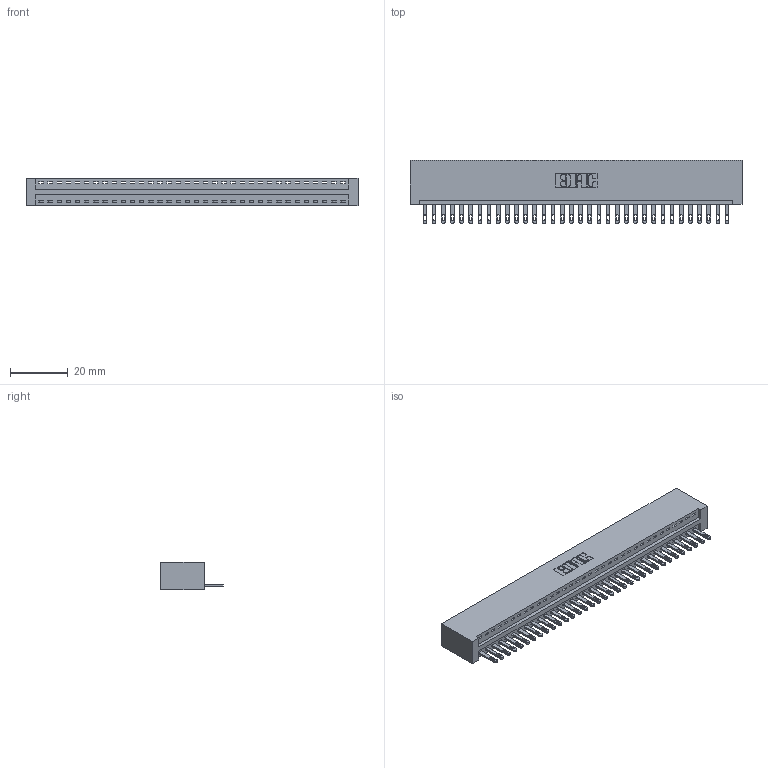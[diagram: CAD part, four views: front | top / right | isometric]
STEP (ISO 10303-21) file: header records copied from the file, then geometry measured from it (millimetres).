
FILE_DESCRIPTION (( 'STEP AP203' ), '1' );
FILE_NAME ('346-034-500-101.STEP', '2022-05-06T20:37:02', ( '' ), ( '' ), 'SwSTEP 2.0', 'SolidWorks 2020', '' );
FILE_SCHEMA (( 'CONFIG_CONTROL_DESIGN' ));
Length unit declared in the file: inch
Products named in the file (3): 346 Part_No Mounting Lugs; 345-292-001_345-293-100; 346-034-500-101
Assembly tree (35 placements, depth 2):
  346-034-500-101
    346 Part_No Mounting Lugs
    345-292-001_345-293-100  x34
Bounding box: 115.19 x 21.84 x 9.4 mm (x, y, z)
Volume: 11541.5 mm3; surface area: 14493.4 mm2
Topology: 35 solids, 35 shells, 1950 faces, 6017 edges, 4010 vertices
Faces by surface type: plane 1228, cylinder 722
Entity records: 21831 total; most frequent: CARTESIAN_POINT 3750, ORIENTED_EDGE 3718, DIRECTION 3315, EDGE_CURVE 1859, LINE 1595, VECTOR 1595, VERTEX_POINT 1238, AXIS2_PLACEMENT_3D 860
